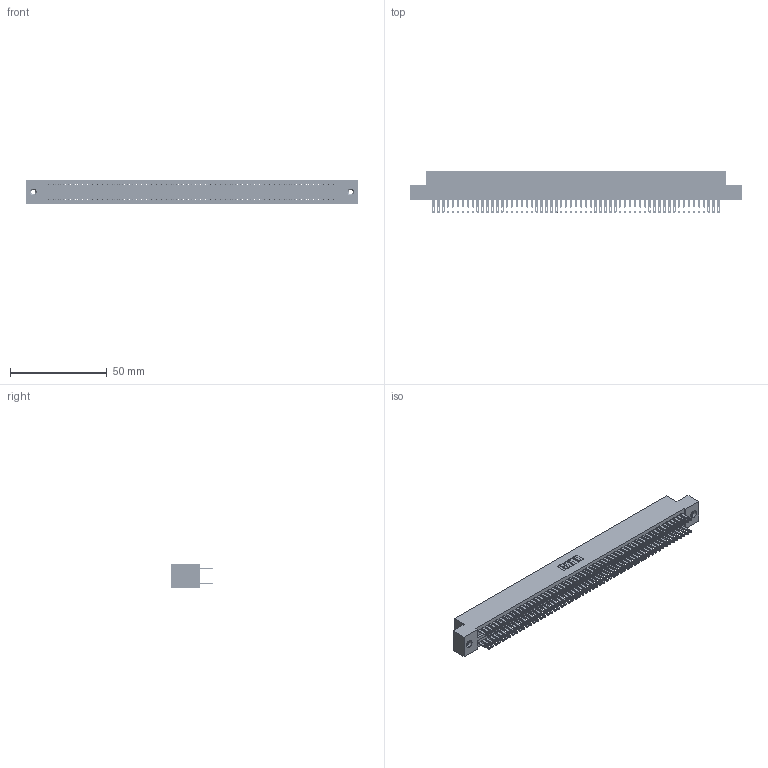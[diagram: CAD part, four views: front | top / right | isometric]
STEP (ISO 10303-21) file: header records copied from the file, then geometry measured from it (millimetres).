
FILE_DESCRIPTION (( 'STEP AP203' ), '1' );
FILE_NAME ('325-118-500-208.STEP', '2020-02-25T08:26:54', ( '' ), ( '' ), 'SwSTEP 2.0', 'SolidWorks 2016', '' );
FILE_SCHEMA (( 'CONFIG_CONTROL_DESIGN' ));
Length unit declared in the file: inch
Products named in the file (4): 345-250-001_345-250-003-102; 325 Part_TI; 325-118-500-208; 325-292-001_325-293-100
Assembly tree (121 placements, depth 2):
  325-118-500-208
    325 Part_TI
    325-292-001_325-293-100  x118
    345-250-001_345-250-003-102  x2
Bounding box: 171.58 x 21.84 x 12.45 mm (x, y, z)
Volume: 22656.5 mm3; surface area: 29073.3 mm2
Topology: 121 solids, 121 shells, 5838 faces, 17793 edges, 11854 vertices
Faces by surface type: plane 3642, cylinder 2180, cone 12, torus 4
Entity records: 36874 total; most frequent: CARTESIAN_POINT 6073, ORIENTED_EDGE 6002, DIRECTION 5191, EDGE_CURVE 3001, LINE 2849, VECTOR 2849, VERTEX_POINT 1996, AXIS2_PLACEMENT_3D 1171
